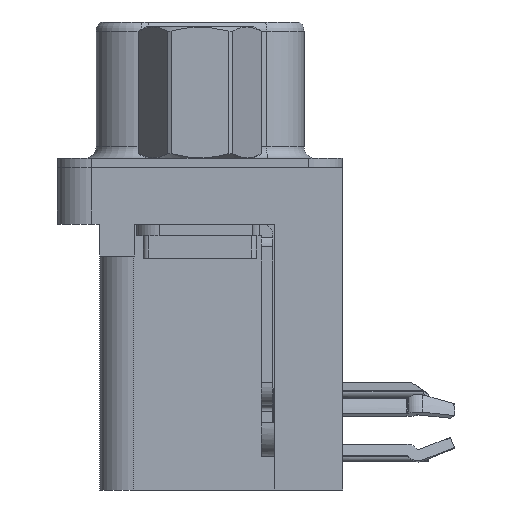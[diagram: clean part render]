
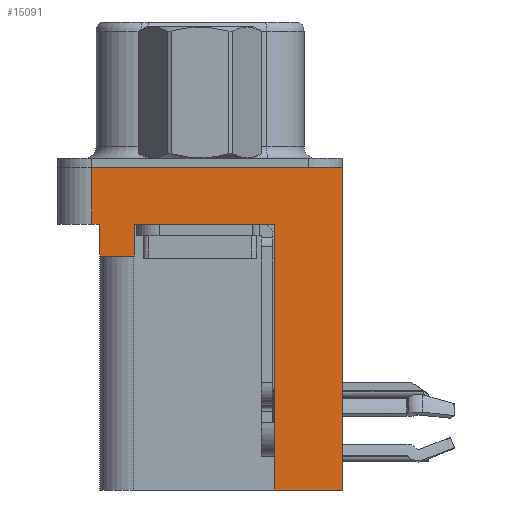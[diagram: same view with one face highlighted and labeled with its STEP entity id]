
A CAD part, left-side view. The second image highlights one B-rep face of the part: STEP entity #15091.
In plain terms, the highlighted planar face has unit normal (-1, 0, 0).
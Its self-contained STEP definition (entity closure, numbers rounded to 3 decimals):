
#339 = DIRECTION ( 'NONE',  ( 0., 0., 1. ) ) ;
#428 = VECTOR ( 'NONE', #3599, 1000. ) ;
#446 = LINE ( 'NONE', #9463, #10689 ) ;
#695 = CARTESIAN_POINT ( 'NONE',  ( -3., -6.275, 0. ) ) ;
#1114 = CARTESIAN_POINT ( 'NONE',  ( -3., 4.425, -3.9 ) ) ;
#2049 = CARTESIAN_POINT ( 'NONE',  ( -3., -3.295, -14.2 ) ) ;
#2312 = ORIENTED_EDGE ( 'NONE', *, *, #19668, .F. ) ;
#2454 = VERTEX_POINT ( 'NONE', #695 ) ;
#3406 = DIRECTION ( 'NONE',  ( 0., -1., 0. ) ) ;
#3599 = DIRECTION ( 'NONE',  ( 0., -1., 0. ) ) ;
#3762 = LINE ( 'NONE', #1114, #13012 ) ;
#4294 = EDGE_CURVE ( 'NONE', #5857, #18457, #18300, .T. ) ;
#4308 = DIRECTION ( 'NONE',  ( 0., 1., 0. ) ) ;
#4937 = CARTESIAN_POINT ( 'NONE',  ( -3., 4.775, -2.5 ) ) ;
#5796 = EDGE_CURVE ( 'NONE', #25878, #13795, #10775, .T. ) ;
#5857 = VERTEX_POINT ( 'NONE', #17391 ) ;
#5906 = DIRECTION ( 'NONE',  ( 0., 0., 1. ) ) ;
#6091 = ORIENTED_EDGE ( 'NONE', *, *, #15833, .F. ) ;
#6345 = DIRECTION ( 'NONE',  ( 0., 0., 1. ) ) ;
#6991 = VECTOR ( 'NONE', #28788, 1000. ) ;
#7328 = CARTESIAN_POINT ( 'NONE',  ( -3., -3.295, -14.2 ) ) ;
#8283 = CARTESIAN_POINT ( 'NONE',  ( -3., -3.295, -2.5 ) ) ;
#8699 = CARTESIAN_POINT ( 'NONE',  ( -3., 4.775, 0. ) ) ;
#9060 = LINE ( 'NONE', #4937, #26694 ) ;
#9463 = CARTESIAN_POINT ( 'NONE',  ( -3., -6.275, -2.5 ) ) ;
#9908 = ORIENTED_EDGE ( 'NONE', *, *, #22828, .T. ) ;
#10158 = DIRECTION ( 'NONE',  ( 0., 0., 1. ) ) ;
#10222 = EDGE_CURVE ( 'NONE', #15148, #23281, #17574, .T. ) ;
#10305 = LINE ( 'NONE', #19156, #16291 ) ;
#10340 = LINE ( 'NONE', #28351, #25521 ) ;
#10689 = VECTOR ( 'NONE', #3406, 1000. ) ;
#10775 = LINE ( 'NONE', #22421, #6991 ) ;
#10827 = CARTESIAN_POINT ( 'NONE',  ( -3., -6.275, 0. ) ) ;
#11247 = VERTEX_POINT ( 'NONE', #15294 ) ;
#11684 = DIRECTION ( 'NONE',  ( 0., 0., 1. ) ) ;
#13012 = VECTOR ( 'NONE', #19396, 1000. ) ;
#13749 = CARTESIAN_POINT ( 'NONE',  ( -3., 4.425, -3.9 ) ) ;
#13795 = VERTEX_POINT ( 'NONE', #8283 ) ;
#13882 = EDGE_CURVE ( 'NONE', #15148, #2454, #10305, .T. ) ;
#14043 = EDGE_CURVE ( 'NONE', #19352, #15072, #9060, .T. ) ;
#14708 = EDGE_CURVE ( 'NONE', #19352, #18457, #446, .T. ) ;
#15072 = VERTEX_POINT ( 'NONE', #8699 ) ;
#15083 = LINE ( 'NONE', #10827, #428 ) ;
#15091 = ADVANCED_FACE ( 'NONE', ( #26992 ), #20474, .T. ) ;
#15141 = VECTOR ( 'NONE', #6345, 1000. ) ;
#15148 = VERTEX_POINT ( 'NONE', #27456 ) ;
#15294 = CARTESIAN_POINT ( 'NONE',  ( -3., 2.895, -3.9 ) ) ;
#15653 = ORIENTED_EDGE ( 'NONE', *, *, #22907, .F. ) ;
#15815 = ORIENTED_EDGE ( 'NONE', *, *, #13882, .T. ) ;
#15833 = EDGE_CURVE ( 'NONE', #11247, #5857, #3762, .T. ) ;
#16168 = VECTOR ( 'NONE', #4308, 1000. ) ;
#16291 = VECTOR ( 'NONE', #10158, 1000. ) ;
#17246 = AXIS2_PLACEMENT_3D ( 'NONE', #19897, #17686, #26704 ) ;
#17391 = CARTESIAN_POINT ( 'NONE',  ( -3., 4.425, -3.9 ) ) ;
#17574 = LINE ( 'NONE', #26596, #16168 ) ;
#17686 = DIRECTION ( 'NONE',  ( -1., 0., 0. ) ) ;
#18300 = LINE ( 'NONE', #13749, #18484 ) ;
#18457 = VERTEX_POINT ( 'NONE', #20081 ) ;
#18484 = VECTOR ( 'NONE', #11684, 1000. ) ;
#19156 = CARTESIAN_POINT ( 'NONE',  ( -3., -6.275, -2.5 ) ) ;
#19352 = VERTEX_POINT ( 'NONE', #26359 ) ;
#19396 = DIRECTION ( 'NONE',  ( 0., 1., 0. ) ) ;
#19668 = EDGE_CURVE ( 'NONE', #15072, #2454, #15083, .T. ) ;
#19897 = CARTESIAN_POINT ( 'NONE',  ( -3., -6.275, -2.5 ) ) ;
#20081 = CARTESIAN_POINT ( 'NONE',  ( -3., 4.425, -2.5 ) ) ;
#20474 = PLANE ( 'NONE',  #17246 ) ;
#21684 = LINE ( 'NONE', #2049, #15141 ) ;
#22421 = CARTESIAN_POINT ( 'NONE',  ( -3., -6.275, -2.5 ) ) ;
#22828 = EDGE_CURVE ( 'NONE', #11247, #25878, #10340, .T. ) ;
#22907 = EDGE_CURVE ( 'NONE', #23281, #13795, #21684, .T. ) ;
#23281 = VERTEX_POINT ( 'NONE', #7328 ) ;
#24158 = ORIENTED_EDGE ( 'NONE', *, *, #5796, .T. ) ;
#24728 = ORIENTED_EDGE ( 'NONE', *, *, #4294, .F. ) ;
#24889 = ORIENTED_EDGE ( 'NONE', *, *, #14708, .T. ) ;
#25521 = VECTOR ( 'NONE', #5906, 1000. ) ;
#25878 = VERTEX_POINT ( 'NONE', #29023 ) ;
#26359 = CARTESIAN_POINT ( 'NONE',  ( -3., 4.775, -2.5 ) ) ;
#26596 = CARTESIAN_POINT ( 'NONE',  ( -3., -3.295, -14.2 ) ) ;
#26694 = VECTOR ( 'NONE', #339, 1000. ) ;
#26704 = DIRECTION ( 'NONE',  ( 0., 0., 1. ) ) ;
#26992 = FACE_OUTER_BOUND ( 'NONE', #28269, .T. ) ;
#27456 = CARTESIAN_POINT ( 'NONE',  ( -3., -6.275, -14.2 ) ) ;
#27855 = ORIENTED_EDGE ( 'NONE', *, *, #14043, .F. ) ;
#28199 = ORIENTED_EDGE ( 'NONE', *, *, #10222, .F. ) ;
#28269 = EDGE_LOOP ( 'NONE', ( #2312, #27855, #24889, #24728, #6091, #9908, #24158, #15653, #28199, #15815 ) ) ;
#28351 = CARTESIAN_POINT ( 'NONE',  ( -3., 2.895, -3.9 ) ) ;
#28788 = DIRECTION ( 'NONE',  ( 0., -1., 0. ) ) ;
#29023 = CARTESIAN_POINT ( 'NONE',  ( -3., 2.895, -2.5 ) ) ;
